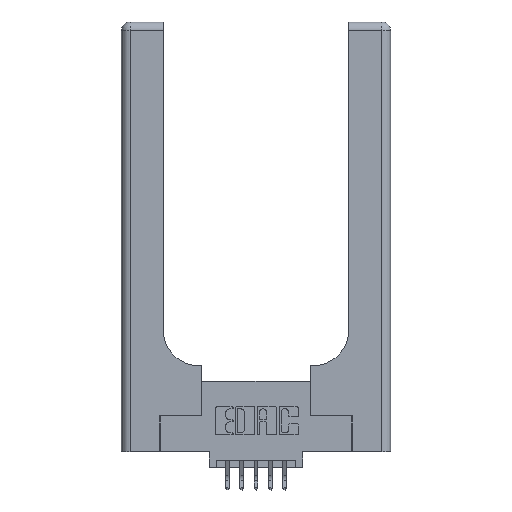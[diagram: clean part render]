
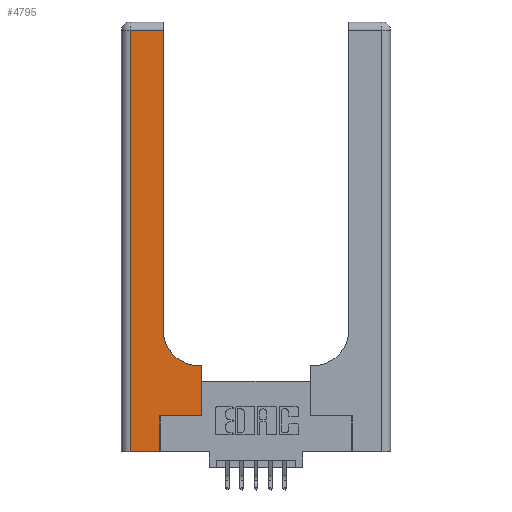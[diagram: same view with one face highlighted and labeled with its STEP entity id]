
A CAD part, top view. The second image highlights one B-rep face of the part: STEP entity #4795.
In plain terms, the highlighted planar face has unit normal (0, 0, 1).
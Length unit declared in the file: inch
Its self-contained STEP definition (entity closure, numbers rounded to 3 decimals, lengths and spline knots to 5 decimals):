
#90 = CARTESIAN_POINT ( 'NONE',  ( 0.5585, 0.25, 0.37 ) ) ;
#144 = DIRECTION ( 'NONE',  ( 1., 0., 0. ) ) ;
#226 = DIRECTION ( 'NONE',  ( -1., 0., 0. ) ) ;
#394 = CARTESIAN_POINT ( 'NONE',  ( 0., 3., 0.37 ) ) ;
#410 = CARTESIAN_POINT ( 'NONE',  ( 0.269, 0., 0.37 ) ) ;
#536 = DIRECTION ( 'NONE',  ( -1., 0., 0. ) ) ;
#694 = EDGE_CURVE ( 'NONE', #6092, #11120, #1567, .T. ) ;
#863 = DIRECTION ( 'NONE',  ( 0., 1., 0. ) ) ;
#996 = VECTOR ( 'NONE', #863, 39.37008 ) ;
#1164 = CARTESIAN_POINT ( 'NONE',  ( 0., 0., 0.37 ) ) ;
#1185 = VERTEX_POINT ( 'NONE', #8288 ) ;
#1200 = DIRECTION ( 'NONE',  ( 0., 1., 0. ) ) ;
#1455 = AXIS2_PLACEMENT_3D ( 'NONE', #394, #10513, #536 ) ;
#1567 = LINE ( 'NONE', #1164, #3707 ) ;
#1878 = VERTEX_POINT ( 'NONE', #3650 ) ;
#1982 = CARTESIAN_POINT ( 'NONE',  ( 0.2915, 0.85, 0.37 ) ) ;
#2076 = VECTOR ( 'NONE', #9701, 39.37008 ) ;
#2402 = ORIENTED_EDGE ( 'NONE', *, *, #11917, .T. ) ;
#2467 = LINE ( 'NONE', #6118, #9439 ) ;
#2689 = CARTESIAN_POINT ( 'NONE',  ( 0.269, 0., 0.37 ) ) ;
#2714 = LINE ( 'NONE', #410, #7960 ) ;
#2791 = VERTEX_POINT ( 'NONE', #1982 ) ;
#2792 = ORIENTED_EDGE ( 'NONE', *, *, #13589, .T. ) ;
#3064 = CARTESIAN_POINT ( 'NONE',  ( 0.06, 2.94, 0.37 ) ) ;
#3500 = VECTOR ( 'NONE', #226, 39.37008 ) ;
#3650 = CARTESIAN_POINT ( 'NONE',  ( 0.5415, 0.6, 0.37 ) ) ;
#3707 = VECTOR ( 'NONE', #10674, 39.37008 ) ;
#3907 = ORIENTED_EDGE ( 'NONE', *, *, #11131, .T. ) ;
#4032 = CARTESIAN_POINT ( 'NONE',  ( 0.06, 0., 0.37 ) ) ;
#4686 = CARTESIAN_POINT ( 'NONE',  ( 0.5415, 0.85, 0.37 ) ) ;
#4795 = ADVANCED_FACE ( 'NONE', ( #13912 ), #12785, .F. ) ;
#4842 = DIRECTION ( 'NONE',  ( -1., 0., 0. ) ) ;
#5052 = ORIENTED_EDGE ( 'NONE', *, *, #12695, .T. ) ;
#5249 = LINE ( 'NONE', #90, #9933 ) ;
#5309 = ORIENTED_EDGE ( 'NONE', *, *, #694, .T. ) ;
#5481 = DIRECTION ( 'NONE',  ( 0., 0., -1. ) ) ;
#6092 = VERTEX_POINT ( 'NONE', #4032 ) ;
#6118 = CARTESIAN_POINT ( 'NONE',  ( 0.269, 0.25, 0.37 ) ) ;
#6356 = EDGE_CURVE ( 'NONE', #1878, #2791, #13361, .T. ) ;
#6960 = CARTESIAN_POINT ( 'NONE',  ( 0., 2.94, 0.37 ) ) ;
#7142 = VECTOR ( 'NONE', #4842, 39.37008 ) ;
#7281 = VERTEX_POINT ( 'NONE', #10058 ) ;
#7359 = CARTESIAN_POINT ( 'NONE',  ( 0.5585, 0.25, 0.37 ) ) ;
#7373 = EDGE_CURVE ( 'NONE', #11120, #14406, #2714, .T. ) ;
#7658 = AXIS2_PLACEMENT_3D ( 'NONE', #4686, #5481, #144 ) ;
#7960 = VECTOR ( 'NONE', #9322, 39.37008 ) ;
#8058 = CARTESIAN_POINT ( 'NONE',  ( 0.2915, 0.6, 0.37 ) ) ;
#8288 = CARTESIAN_POINT ( 'NONE',  ( 0.2915, 2.94, 0.37 ) ) ;
#8647 = EDGE_LOOP ( 'NONE', ( #2792, #5052, #10375, #5309, #13972, #3907, #2402, #11200, #13996 ) ) ;
#9322 = DIRECTION ( 'NONE',  ( 0., 1., 0. ) ) ;
#9439 = VECTOR ( 'NONE', #13942, 39.37008 ) ;
#9563 = LINE ( 'NONE', #10878, #2076 ) ;
#9701 = DIRECTION ( 'NONE',  ( 0., -1., 0. ) ) ;
#9933 = VECTOR ( 'NONE', #1200, 39.37008 ) ;
#9973 = VERTEX_POINT ( 'NONE', #3064 ) ;
#10058 = CARTESIAN_POINT ( 'NONE',  ( 0.5585, 0.6, 0.37 ) ) ;
#10248 = LINE ( 'NONE', #8058, #7142 ) ;
#10375 = ORIENTED_EDGE ( 'NONE', *, *, #12395, .T. ) ;
#10513 = DIRECTION ( 'NONE',  ( 0., 0., -1. ) ) ;
#10608 = LINE ( 'NONE', #6960, #3500 ) ;
#10674 = DIRECTION ( 'NONE',  ( 1., 0., 0. ) ) ;
#10878 = CARTESIAN_POINT ( 'NONE',  ( 0.06, 3., 0.37 ) ) ;
#11120 = VERTEX_POINT ( 'NONE', #2689 ) ;
#11131 = EDGE_CURVE ( 'NONE', #14406, #12749, #2467, .T. ) ;
#11200 = ORIENTED_EDGE ( 'NONE', *, *, #12612, .T. ) ;
#11679 = CARTESIAN_POINT ( 'NONE',  ( 0.269, 0.25, 0.37 ) ) ;
#11917 = EDGE_CURVE ( 'NONE', #12749, #7281, #5249, .T. ) ;
#12395 = EDGE_CURVE ( 'NONE', #9973, #6092, #9563, .T. ) ;
#12612 = EDGE_CURVE ( 'NONE', #7281, #1878, #10248, .T. ) ;
#12695 = EDGE_CURVE ( 'NONE', #1185, #9973, #10608, .T. ) ;
#12749 = VERTEX_POINT ( 'NONE', #7359 ) ;
#12785 = PLANE ( 'NONE',  #1455 ) ;
#13182 = CARTESIAN_POINT ( 'NONE',  ( 0.2915, 3., 0.37 ) ) ;
#13193 = LINE ( 'NONE', #13182, #996 ) ;
#13361 = CIRCLE ( 'NONE', #7658, 0.25 ) ;
#13589 = EDGE_CURVE ( 'NONE', #2791, #1185, #13193, .T. ) ;
#13912 = FACE_OUTER_BOUND ( 'NONE', #8647, .T. ) ;
#13942 = DIRECTION ( 'NONE',  ( 1., 0., 0. ) ) ;
#13972 = ORIENTED_EDGE ( 'NONE', *, *, #7373, .T. ) ;
#13996 = ORIENTED_EDGE ( 'NONE', *, *, #6356, .T. ) ;
#14406 = VERTEX_POINT ( 'NONE', #11679 ) ;
